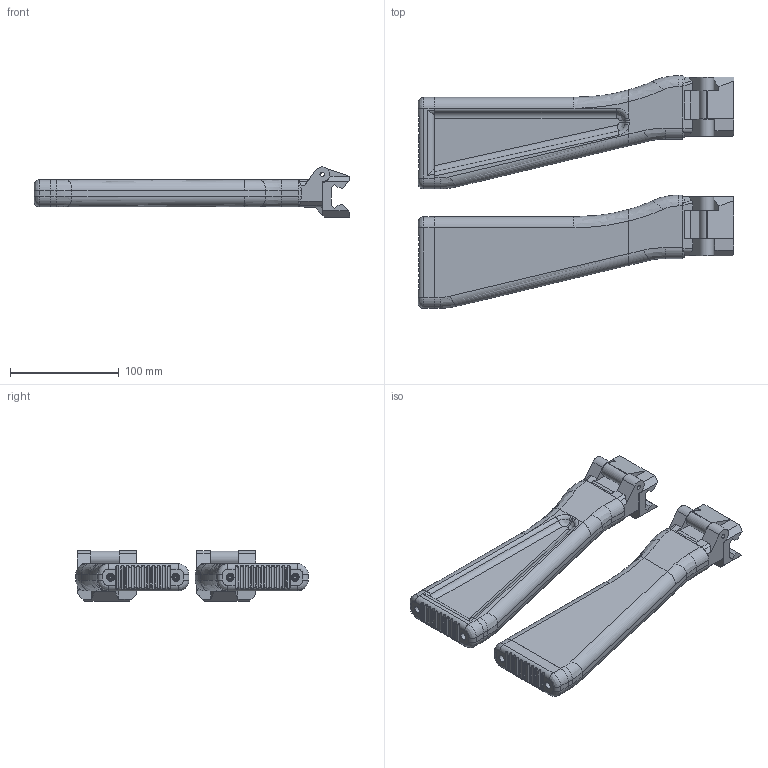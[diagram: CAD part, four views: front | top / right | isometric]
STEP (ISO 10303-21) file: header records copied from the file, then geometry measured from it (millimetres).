
FILE_DESCRIPTION(/* description */ (''),/* implementation_level */ '2;1');
FILE_NAME(/* name */ 'MP5 A3 STOCK.stp',/* time_stamp */ '2021-01-30T10:41:22+02:00',/* author */ (''),/* organization */ (''),/* preprocessor_version */ 'ST-DEVELOPER v15.2',/* originating_system */ 'Autodesk Translator Framework v2.0.0.5431',/* authorisation */ '');
FILE_SCHEMA (('AUTOMOTIVE_DESIGN { 1 0 10303 214 3 1 1 }'));
Length unit declared in the file: centimetre
Products named in the file (1): unpublished stocks
Bounding box: 290.65 x 214.31 x 46.3 mm (x, y, z)
Volume: 535722.2 mm3; surface area: 193080.6 mm2
Topology: 8 solids, 8 shells, 703 faces, 1889 edges, 1214 vertices
Faces by surface type: plane 267, cylinder 210, bspline 190, cone 22, torus 14
Full cylindrical faces by diameter (mm): 3 x2, 3.5 x4, 4 x6, 6.5 x4, 12.1 x2, 20.5 x2
Entity records: 30594 total; most frequent: CARTESIAN_POINT 13901, ORIENTED_EDGE 3694, DIRECTION 3163, EDGE_CURVE 1847, VERTEX_POINT 1208, AXIS2_PLACEMENT_3D 1124, LINE 915, VECTOR 915
